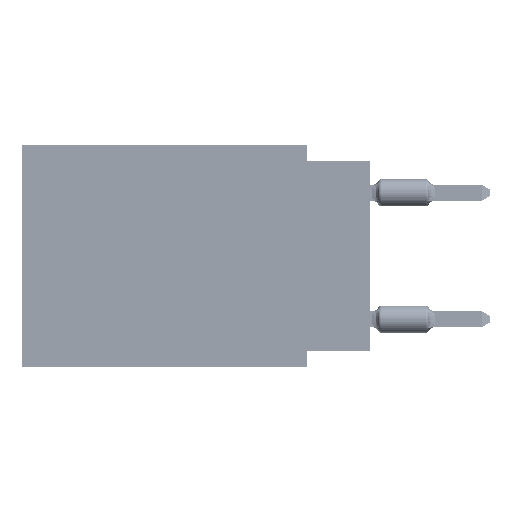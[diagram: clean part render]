
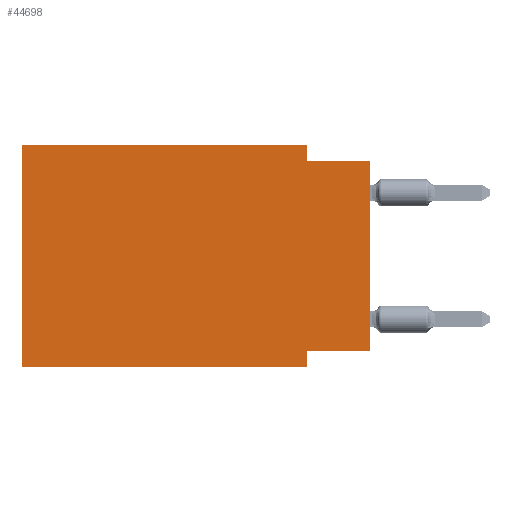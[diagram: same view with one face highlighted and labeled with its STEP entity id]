
A CAD part, left-side view. The second image highlights one B-rep face of the part: STEP entity #44698.
In plain terms, the highlighted planar face has unit normal (-1, 0, 0).
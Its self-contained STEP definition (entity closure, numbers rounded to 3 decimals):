
#523 = VERTEX_POINT ( 'NONE', #8853 ) ;
#2045 = ORIENTED_EDGE ( 'NONE', *, *, #67059, .F. ) ;
#4294 = CARTESIAN_POINT ( 'NONE',  ( 0., 2.54, 0. ) ) ;
#4560 = VERTEX_POINT ( 'NONE', #15484 ) ;
#7981 = LINE ( 'NONE', #45719, #22282 ) ;
#8853 = CARTESIAN_POINT ( 'NONE',  ( 0., 0., -8.255 ) ) ;
#9828 = VECTOR ( 'NONE', #77585, 1000. ) ;
#10793 = FACE_OUTER_BOUND ( 'NONE', #29842, .T. ) ;
#12237 = DIRECTION ( 'NONE',  ( 1., 0., 0. ) ) ;
#12649 = ORIENTED_EDGE ( 'NONE', *, *, #45372, .T. ) ;
#13107 = VECTOR ( 'NONE', #35155, 1000. ) ;
#13203 = VECTOR ( 'NONE', #14120, 1000. ) ;
#14120 = DIRECTION ( 'NONE',  ( 0., 0., 1. ) ) ;
#15453 = LINE ( 'NONE', #66787, #36961 ) ;
#15484 = CARTESIAN_POINT ( 'NONE',  ( 0., 2.54, -8.255 ) ) ;
#16801 = ORIENTED_EDGE ( 'NONE', *, *, #67373, .T. ) ;
#17627 = ORIENTED_EDGE ( 'NONE', *, *, #43435, .F. ) ;
#19516 = AXIS2_PLACEMENT_3D ( 'NONE', #71304, #12237, #85360 ) ;
#22228 = DIRECTION ( 'NONE',  ( 0., 0., -1. ) ) ;
#22282 = VECTOR ( 'NONE', #60716, 1000. ) ;
#23011 = VERTEX_POINT ( 'NONE', #4294 ) ;
#26404 = LINE ( 'NONE', #47217, #78343 ) ;
#28175 = PLANE ( 'NONE',  #19516 ) ;
#29842 = EDGE_LOOP ( 'NONE', ( #16801, #77569, #31514, #17627, #55852, #12649, #2045, #46950 ) ) ;
#31514 = ORIENTED_EDGE ( 'NONE', *, *, #59684, .F. ) ;
#31593 = LINE ( 'NONE', #39332, #9828 ) ;
#31654 = VECTOR ( 'NONE', #72311, 1000. ) ;
#33416 = VECTOR ( 'NONE', #66263, 1000. ) ;
#35155 = DIRECTION ( 'NONE',  ( 0., 1., 0. ) ) ;
#35960 = LINE ( 'NONE', #79550, #31654 ) ;
#36179 = CARTESIAN_POINT ( 'NONE',  ( 0., 2.54, -8.89 ) ) ;
#36720 = LINE ( 'NONE', #88531, #33416 ) ;
#36961 = VECTOR ( 'NONE', #22228, 1000. ) ;
#39332 = CARTESIAN_POINT ( 'NONE',  ( 0., 2.54, -8.89 ) ) ;
#41598 = CARTESIAN_POINT ( 'NONE',  ( 0., 13.97, -8.89 ) ) ;
#43435 = EDGE_CURVE ( 'NONE', #76276, #23011, #36720, .T. ) ;
#44698 = ADVANCED_FACE ( 'NONE', ( #10793 ), #28175, .F. ) ;
#45372 = EDGE_CURVE ( 'NONE', #55656, #81188, #26404, .T. ) ;
#45719 = CARTESIAN_POINT ( 'NONE',  ( 0., 0., -0.635 ) ) ;
#46950 = ORIENTED_EDGE ( 'NONE', *, *, #83607, .F. ) ;
#47217 = CARTESIAN_POINT ( 'NONE',  ( 0., 13.97, -8.89 ) ) ;
#47771 = EDGE_CURVE ( 'NONE', #55656, #76276, #35960, .T. ) ;
#48144 = CARTESIAN_POINT ( 'NONE',  ( 0., 0., -0.635 ) ) ;
#50123 = CARTESIAN_POINT ( 'NONE',  ( 0., 0., -8.255 ) ) ;
#55656 = VERTEX_POINT ( 'NONE', #41598 ) ;
#55852 = ORIENTED_EDGE ( 'NONE', *, *, #47771, .F. ) ;
#56934 = LINE ( 'NONE', #50123, #13107 ) ;
#59100 = LINE ( 'NONE', #73664, #13203 ) ;
#59684 = EDGE_CURVE ( 'NONE', #23011, #94657, #15453, .T. ) ;
#60716 = DIRECTION ( 'NONE',  ( 0., -1., 0. ) ) ;
#63151 = VERTEX_POINT ( 'NONE', #48144 ) ;
#66263 = DIRECTION ( 'NONE',  ( 0., -1., 0. ) ) ;
#66787 = CARTESIAN_POINT ( 'NONE',  ( 0., 2.54, 0. ) ) ;
#67059 = EDGE_CURVE ( 'NONE', #4560, #81188, #31593, .T. ) ;
#67152 = CARTESIAN_POINT ( 'NONE',  ( 0., 13.97, 0. ) ) ;
#67373 = EDGE_CURVE ( 'NONE', #523, #63151, #59100, .T. ) ;
#71304 = CARTESIAN_POINT ( 'NONE',  ( 0., 13.97, 0. ) ) ;
#72311 = DIRECTION ( 'NONE',  ( 0., 0., 1. ) ) ;
#73664 = CARTESIAN_POINT ( 'NONE',  ( 0., 0., 0. ) ) ;
#76276 = VERTEX_POINT ( 'NONE', #67152 ) ;
#76758 = EDGE_CURVE ( 'NONE', #94657, #63151, #7981, .T. ) ;
#77569 = ORIENTED_EDGE ( 'NONE', *, *, #76758, .F. ) ;
#77585 = DIRECTION ( 'NONE',  ( 0., 0., -1. ) ) ;
#78343 = VECTOR ( 'NONE', #84039, 1000. ) ;
#79550 = CARTESIAN_POINT ( 'NONE',  ( 0., 13.97, 0. ) ) ;
#81188 = VERTEX_POINT ( 'NONE', #36179 ) ;
#81816 = CARTESIAN_POINT ( 'NONE',  ( 0., 2.54, -0.635 ) ) ;
#83607 = EDGE_CURVE ( 'NONE', #523, #4560, #56934, .T. ) ;
#84039 = DIRECTION ( 'NONE',  ( 0., -1., 0. ) ) ;
#85360 = DIRECTION ( 'NONE',  ( 0., 0., -1. ) ) ;
#88531 = CARTESIAN_POINT ( 'NONE',  ( 0., 13.97, 0. ) ) ;
#94657 = VERTEX_POINT ( 'NONE', #81816 ) ;
